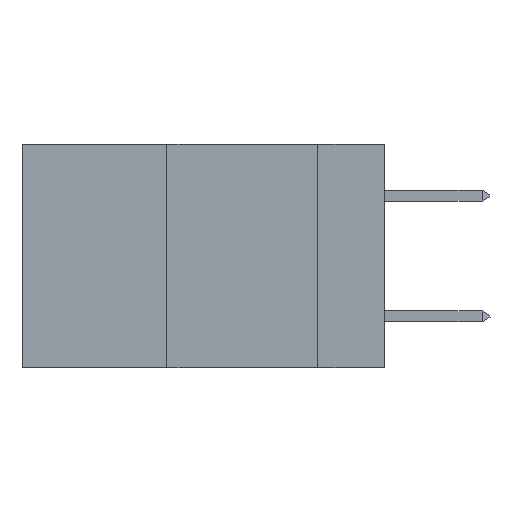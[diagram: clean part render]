
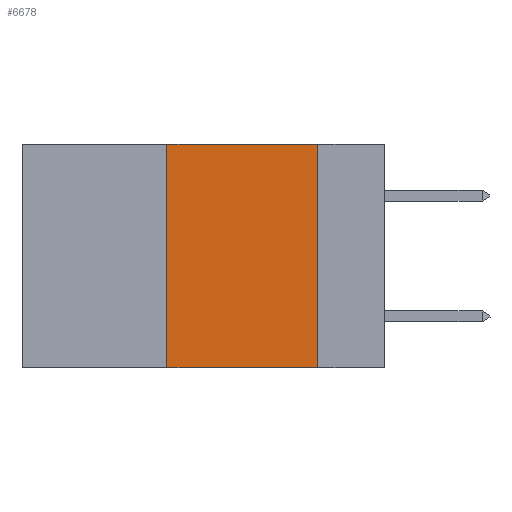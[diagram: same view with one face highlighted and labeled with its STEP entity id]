
A CAD part, left-side view. The second image highlights one B-rep face of the part: STEP entity #6678.
In plain terms, the highlighted planar face has unit normal (-1, 0, 0).
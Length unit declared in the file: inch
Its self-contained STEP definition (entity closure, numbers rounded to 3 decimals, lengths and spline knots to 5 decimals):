
#286 = CARTESIAN_POINT ( 'NONE',  ( 0., 0.36, 0. ) ) ;
#651 = DIRECTION ( 'NONE',  ( 0., -1., 0. ) ) ;
#1968 = DIRECTION ( 'NONE',  ( 0., 0., 1. ) ) ;
#2035 = CARTESIAN_POINT ( 'NONE',  ( 0., 0.36, 0. ) ) ;
#3156 = CARTESIAN_POINT ( 'NONE',  ( 0., 0.11, 0. ) ) ;
#3668 = VECTOR ( 'NONE', #1968, 39.37008 ) ;
#4029 = EDGE_CURVE ( 'NONE', #16997, #6487, #19395, .T. ) ;
#4819 = DIRECTION ( 'NONE',  ( 0., 0., -1. ) ) ;
#5217 = CARTESIAN_POINT ( 'NONE',  ( 0., 0.11, -0.37 ) ) ;
#5622 = CARTESIAN_POINT ( 'NONE',  ( 0., 0.6, 0. ) ) ;
#6069 = VERTEX_POINT ( 'NONE', #12501 ) ;
#6241 = DIRECTION ( 'NONE',  ( 1., 0., 0. ) ) ;
#6363 = EDGE_LOOP ( 'NONE', ( #7220, #7243, #8248, #8479 ) ) ;
#6487 = VERTEX_POINT ( 'NONE', #9022 ) ;
#6678 = ADVANCED_FACE ( 'NONE', ( #14070 ), #14279, .F. ) ;
#7220 = ORIENTED_EDGE ( 'NONE', *, *, #13892, .F. ) ;
#7243 = ORIENTED_EDGE ( 'NONE', *, *, #4029, .F. ) ;
#8051 = LINE ( 'NONE', #286, #3668 ) ;
#8248 = ORIENTED_EDGE ( 'NONE', *, *, #16971, .F. ) ;
#8479 = ORIENTED_EDGE ( 'NONE', *, *, #18382, .T. ) ;
#9022 = CARTESIAN_POINT ( 'NONE',  ( 0., 0.11, 0. ) ) ;
#9119 = DIRECTION ( 'NONE',  ( 0., -1., 0. ) ) ;
#9305 = VECTOR ( 'NONE', #9119, 39.37008 ) ;
#9735 = LINE ( 'NONE', #3156, #17575 ) ;
#10310 = LINE ( 'NONE', #12290, #9305 ) ;
#10866 = AXIS2_PLACEMENT_3D ( 'NONE', #15803, #6241, #17350 ) ;
#11105 = VECTOR ( 'NONE', #651, 39.37008 ) ;
#12290 = CARTESIAN_POINT ( 'NONE',  ( 0., 0.6, -0.37 ) ) ;
#12501 = CARTESIAN_POINT ( 'NONE',  ( 0., 0.36, -0.37 ) ) ;
#13892 = EDGE_CURVE ( 'NONE', #6487, #19499, #9735, .T. ) ;
#14070 = FACE_OUTER_BOUND ( 'NONE', #6363, .T. ) ;
#14279 = PLANE ( 'NONE',  #10866 ) ;
#15803 = CARTESIAN_POINT ( 'NONE',  ( 0., 0.6, 0. ) ) ;
#16971 = EDGE_CURVE ( 'NONE', #6069, #16997, #8051, .T. ) ;
#16997 = VERTEX_POINT ( 'NONE', #2035 ) ;
#17350 = DIRECTION ( 'NONE',  ( 0., 0., -1. ) ) ;
#17575 = VECTOR ( 'NONE', #4819, 39.37008 ) ;
#18382 = EDGE_CURVE ( 'NONE', #6069, #19499, #10310, .T. ) ;
#19395 = LINE ( 'NONE', #5622, #11105 ) ;
#19499 = VERTEX_POINT ( 'NONE', #5217 ) ;
